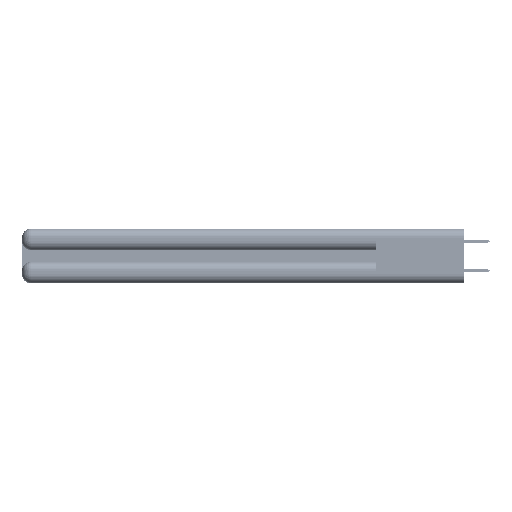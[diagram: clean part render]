
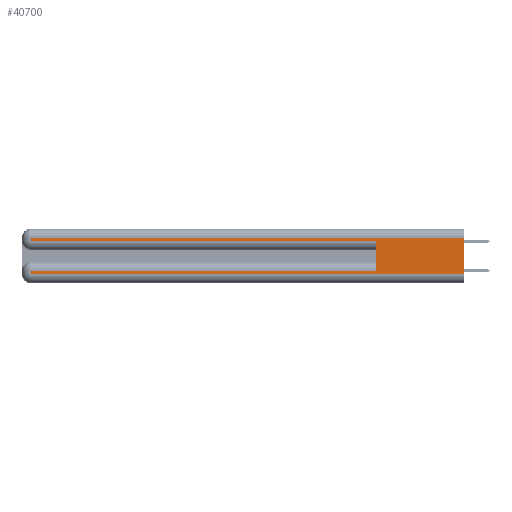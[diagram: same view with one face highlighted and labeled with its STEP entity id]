
A CAD part, left-side view. The second image highlights one B-rep face of the part: STEP entity #40700.
In plain terms, the highlighted planar face has unit normal (-1, 0, 0).
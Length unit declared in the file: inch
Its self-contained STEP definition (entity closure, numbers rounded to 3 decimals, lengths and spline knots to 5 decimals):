
#222 = EDGE_CURVE ( 'NONE', #15402, #40421, #23372, .T. ) ;
#445 = VECTOR ( 'NONE', #14928, 39.37008 ) ;
#967 = CARTESIAN_POINT ( 'NONE',  ( 0., 0.6, 0.085 ) ) ;
#971 = CARTESIAN_POINT ( 'NONE',  ( 0., 0., 0.06 ) ) ;
#1755 = VERTEX_POINT ( 'NONE', #967 ) ;
#2467 = ORIENTED_EDGE ( 'NONE', *, *, #11144, .T. ) ;
#3812 = CARTESIAN_POINT ( 'NONE',  ( 0., 2.94, 0.31 ) ) ;
#4081 = ORIENTED_EDGE ( 'NONE', *, *, #30361, .T. ) ;
#4237 = VECTOR ( 'NONE', #49388, 39.37008 ) ;
#4901 = CARTESIAN_POINT ( 'NONE',  ( 0., 2.94, 0.06 ) ) ;
#5449 = DIRECTION ( 'NONE',  ( 0., 0., -1. ) ) ;
#5625 = EDGE_CURVE ( 'NONE', #36147, #15402, #39090, .T. ) ;
#7480 = VERTEX_POINT ( 'NONE', #3812 ) ;
#8107 = CARTESIAN_POINT ( 'NONE',  ( 0., 0., 0.06 ) ) ;
#8313 = VERTEX_POINT ( 'NONE', #12182 ) ;
#9196 = ORIENTED_EDGE ( 'NONE', *, *, #26960, .T. ) ;
#11144 = EDGE_CURVE ( 'NONE', #8313, #48957, #40011, .T. ) ;
#11333 = VECTOR ( 'NONE', #41954, 39.37008 ) ;
#12182 = CARTESIAN_POINT ( 'NONE',  ( 0., 2.94, 0.285 ) ) ;
#13126 = LINE ( 'NONE', #46147, #16132 ) ;
#13784 = EDGE_CURVE ( 'NONE', #1755, #48957, #13126, .T. ) ;
#14870 = AXIS2_PLACEMENT_3D ( 'NONE', #21392, #25101, #48043 ) ;
#14928 = DIRECTION ( 'NONE',  ( 0., -1., 0. ) ) ;
#15402 = VERTEX_POINT ( 'NONE', #4901 ) ;
#16132 = VECTOR ( 'NONE', #28101, 39.37008 ) ;
#16415 = VECTOR ( 'NONE', #17167, 39.37008 ) ;
#17167 = DIRECTION ( 'NONE',  ( 0., -1., 0. ) ) ;
#18210 = ORIENTED_EDGE ( 'NONE', *, *, #5625, .T. ) ;
#18422 = VECTOR ( 'NONE', #26117, 39.37008 ) ;
#19398 = VECTOR ( 'NONE', #46221, 39.37008 ) ;
#20439 = CARTESIAN_POINT ( 'NONE',  ( 0., 0., 0.37 ) ) ;
#20552 = ORIENTED_EDGE ( 'NONE', *, *, #26474, .T. ) ;
#20861 = CARTESIAN_POINT ( 'NONE',  ( 0., 0., 0.285 ) ) ;
#21392 = CARTESIAN_POINT ( 'NONE',  ( 0., 0., 0.37 ) ) ;
#22649 = CARTESIAN_POINT ( 'NONE',  ( 0., 0., 0.31 ) ) ;
#22932 = LINE ( 'NONE', #49228, #4237 ) ;
#23372 = LINE ( 'NONE', #971, #445 ) ;
#25101 = DIRECTION ( 'NONE',  ( 1., 0., 0. ) ) ;
#25635 = VERTEX_POINT ( 'NONE', #22649 ) ;
#26117 = DIRECTION ( 'NONE',  ( 0., 1., 0. ) ) ;
#26291 = CARTESIAN_POINT ( 'NONE',  ( 0., 0., 0.085 ) ) ;
#26474 = EDGE_CURVE ( 'NONE', #7480, #8313, #38149, .T. ) ;
#26960 = EDGE_CURVE ( 'NONE', #25635, #7480, #22932, .T. ) ;
#28101 = DIRECTION ( 'NONE',  ( 0., 0., 1. ) ) ;
#28710 = PLANE ( 'NONE',  #14870 ) ;
#29561 = ORIENTED_EDGE ( 'NONE', *, *, #13784, .F. ) ;
#29924 = LINE ( 'NONE', #26291, #18422 ) ;
#30361 = EDGE_CURVE ( 'NONE', #1755, #36147, #29924, .T. ) ;
#32122 = ORIENTED_EDGE ( 'NONE', *, *, #222, .T. ) ;
#33718 = FACE_OUTER_BOUND ( 'NONE', #35138, .T. ) ;
#35138 = EDGE_LOOP ( 'NONE', ( #45581, #9196, #20552, #2467, #29561, #4081, #18210, #32122 ) ) ;
#36147 = VERTEX_POINT ( 'NONE', #46156 ) ;
#38149 = LINE ( 'NONE', #46563, #19398 ) ;
#38578 = CARTESIAN_POINT ( 'NONE',  ( 0., 2.94, 0.37 ) ) ;
#39090 = LINE ( 'NONE', #38578, #11333 ) ;
#40011 = LINE ( 'NONE', #20861, #16415 ) ;
#40255 = LINE ( 'NONE', #20439, #46829 ) ;
#40421 = VERTEX_POINT ( 'NONE', #8107 ) ;
#40700 = ADVANCED_FACE ( 'NONE', ( #33718 ), #28710, .F. ) ;
#41936 = EDGE_CURVE ( 'NONE', #25635, #40421, #40255, .T. ) ;
#41954 = DIRECTION ( 'NONE',  ( 0., 0., -1. ) ) ;
#45581 = ORIENTED_EDGE ( 'NONE', *, *, #41936, .F. ) ;
#46147 = CARTESIAN_POINT ( 'NONE',  ( 0., 0.6, 0.145 ) ) ;
#46156 = CARTESIAN_POINT ( 'NONE',  ( 0., 2.94, 0.085 ) ) ;
#46221 = DIRECTION ( 'NONE',  ( 0., 0., -1. ) ) ;
#46563 = CARTESIAN_POINT ( 'NONE',  ( 0., 2.94, 0.37 ) ) ;
#46829 = VECTOR ( 'NONE', #5449, 39.37008 ) ;
#48043 = DIRECTION ( 'NONE',  ( 0., 0., -1. ) ) ;
#48957 = VERTEX_POINT ( 'NONE', #49978 ) ;
#49228 = CARTESIAN_POINT ( 'NONE',  ( 0., 0., 0.31 ) ) ;
#49388 = DIRECTION ( 'NONE',  ( 0., 1., 0. ) ) ;
#49978 = CARTESIAN_POINT ( 'NONE',  ( 0., 0.6, 0.285 ) ) ;
